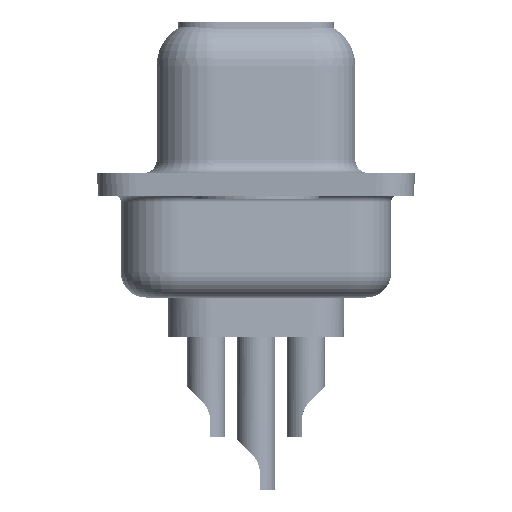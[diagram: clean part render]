
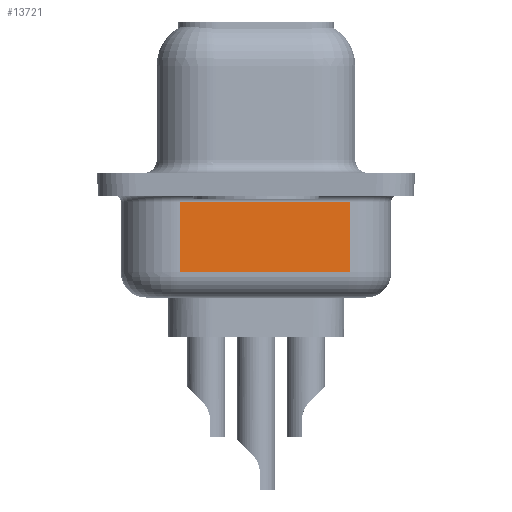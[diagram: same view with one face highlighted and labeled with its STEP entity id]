
A CAD part, left-side view. The second image highlights one B-rep face of the part: STEP entity #13721.
In plain terms, the highlighted planar face has unit normal (-0.985, -0.174, 0).
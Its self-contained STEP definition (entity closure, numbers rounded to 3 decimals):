
#732 = EDGE_CURVE ( 'NONE', #21317, #31845, #4821, .T. ) ;
#2419 = VECTOR ( 'NONE', #12859, 1000. ) ;
#3525 = ORIENTED_EDGE ( 'NONE', *, *, #19489, .F. ) ;
#4796 = ORIENTED_EDGE ( 'NONE', *, *, #5119, .T. ) ;
#4821 = LINE ( 'NONE', #33848, #15088 ) ;
#5119 = EDGE_CURVE ( 'NONE', #31845, #32387, #26419, .T. ) ;
#6995 = LINE ( 'NONE', #28205, #30037 ) ;
#7647 = CARTESIAN_POINT ( 'NONE',  ( 4.191, -3.722, -4.5 ) ) ;
#7864 = VECTOR ( 'NONE', #28656, 1000. ) ;
#8032 = EDGE_LOOP ( 'NONE', ( #3525, #29543, #4796, #25437 ) ) ;
#10372 = VERTEX_POINT ( 'NONE', #29788 ) ;
#11264 = DIRECTION ( 'NONE',  ( 0.985, 0.174, 0. ) ) ;
#12178 = CARTESIAN_POINT ( 'NONE',  ( 3., 3.028, -4.5 ) ) ;
#12859 = DIRECTION ( 'NONE',  ( 0., 0., 1. ) ) ;
#13675 = CARTESIAN_POINT ( 'NONE',  ( 3., 3.028, -4.5 ) ) ;
#13697 = FACE_OUTER_BOUND ( 'NONE', #8032, .T. ) ;
#13721 = ADVANCED_FACE ( 'NONE', ( #13697 ), #24472, .F. ) ;
#14180 = CARTESIAN_POINT ( 'NONE',  ( 4.191, -3.722, -3.5 ) ) ;
#15088 = VECTOR ( 'NONE', #23410, 1000. ) ;
#15129 = CARTESIAN_POINT ( 'NONE',  ( 4.191, -3.722, -0.7 ) ) ;
#15289 = LINE ( 'NONE', #12178, #7864 ) ;
#18620 = DIRECTION ( 'NONE',  ( -0.174, 0.985, 0. ) ) ;
#19489 = EDGE_CURVE ( 'NONE', #21317, #10372, #15289, .T. ) ;
#19764 = CARTESIAN_POINT ( 'NONE',  ( 3., 3.028, -3.5 ) ) ;
#21317 = VERTEX_POINT ( 'NONE', #19764 ) ;
#23410 = DIRECTION ( 'NONE',  ( 0.174, -0.985, 0. ) ) ;
#24472 = PLANE ( 'NONE',  #27923 ) ;
#25437 = ORIENTED_EDGE ( 'NONE', *, *, #27151, .T. ) ;
#26419 = LINE ( 'NONE', #7647, #2419 ) ;
#27151 = EDGE_CURVE ( 'NONE', #32387, #10372, #6995, .T. ) ;
#27923 = AXIS2_PLACEMENT_3D ( 'NONE', #13675, #11264, #29843 ) ;
#28205 = CARTESIAN_POINT ( 'NONE',  ( 3., 3.028, -0.7 ) ) ;
#28656 = DIRECTION ( 'NONE',  ( 0., 0., 1. ) ) ;
#29543 = ORIENTED_EDGE ( 'NONE', *, *, #732, .T. ) ;
#29788 = CARTESIAN_POINT ( 'NONE',  ( 3., 3.028, -0.7 ) ) ;
#29843 = DIRECTION ( 'NONE',  ( -0.174, 0.985, 0. ) ) ;
#30037 = VECTOR ( 'NONE', #18620, 1000. ) ;
#31845 = VERTEX_POINT ( 'NONE', #14180 ) ;
#32387 = VERTEX_POINT ( 'NONE', #15129 ) ;
#33848 = CARTESIAN_POINT ( 'NONE',  ( 3., 3.028, -3.5 ) ) ;
